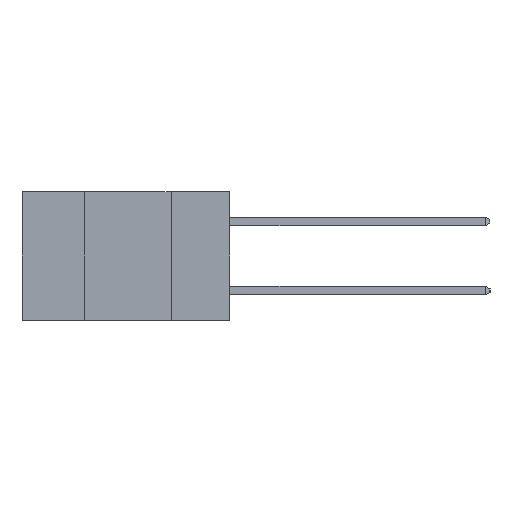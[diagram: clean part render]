
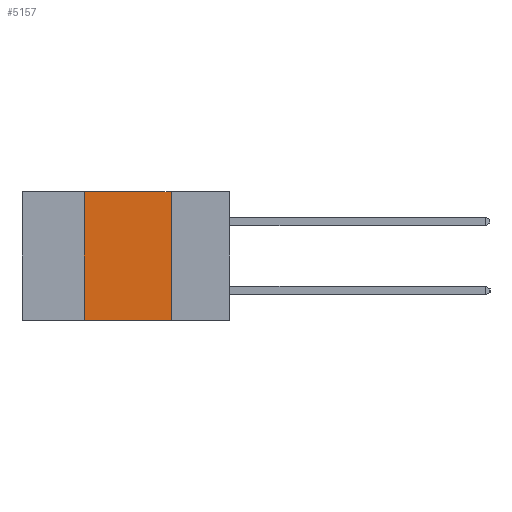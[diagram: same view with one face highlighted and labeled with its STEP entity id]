
A CAD part, left-side view. The second image highlights one B-rep face of the part: STEP entity #5157.
In plain terms, the highlighted planar face has unit normal (-1, 0, 0).
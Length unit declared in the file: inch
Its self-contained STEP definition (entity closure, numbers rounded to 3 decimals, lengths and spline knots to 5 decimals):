
#40 = VERTEX_POINT ( 'NONE', #924 ) ;
#129 = EDGE_LOOP ( 'NONE', ( #3457, #1389, #6023, #1905 ) ) ;
#153 = DIRECTION ( 'NONE',  ( 0., -1., 0. ) ) ;
#199 = EDGE_CURVE ( 'NONE', #40, #6996, #1399, .T. ) ;
#924 = CARTESIAN_POINT ( 'NONE',  ( 0., 0.42, -0.37 ) ) ;
#1389 = ORIENTED_EDGE ( 'NONE', *, *, #9285, .F. ) ;
#1399 = LINE ( 'NONE', #3544, #8061 ) ;
#1658 = FACE_OUTER_BOUND ( 'NONE', #129, .T. ) ;
#1905 = ORIENTED_EDGE ( 'NONE', *, *, #6054, .T. ) ;
#2458 = PLANE ( 'NONE',  #2797 ) ;
#2739 = CARTESIAN_POINT ( 'NONE',  ( 0., 0.17, -0.37 ) ) ;
#2797 = AXIS2_PLACEMENT_3D ( 'NONE', #7676, #8531, #3378 ) ;
#2953 = DIRECTION ( 'NONE',  ( 0., 0., 1. ) ) ;
#3378 = DIRECTION ( 'NONE',  ( 0., 0., -1. ) ) ;
#3457 = ORIENTED_EDGE ( 'NONE', *, *, #4736, .F. ) ;
#3544 = CARTESIAN_POINT ( 'NONE',  ( 0., 0.42, -0.37 ) ) ;
#3731 = CARTESIAN_POINT ( 'NONE',  ( 0., 0.6, -0.37 ) ) ;
#3850 = LINE ( 'NONE', #8376, #10306 ) ;
#4030 = LINE ( 'NONE', #5407, #10489 ) ;
#4540 = DIRECTION ( 'NONE',  ( 0., 0., -1. ) ) ;
#4736 = EDGE_CURVE ( 'NONE', #5844, #9064, #4030, .T. ) ;
#5157 = ADVANCED_FACE ( 'NONE', ( #1658 ), #2458, .F. ) ;
#5407 = CARTESIAN_POINT ( 'NONE',  ( 0., 0.17, -0.37 ) ) ;
#5806 = DIRECTION ( 'NONE',  ( 0., -1., 0. ) ) ;
#5844 = VERTEX_POINT ( 'NONE', #6013 ) ;
#6013 = CARTESIAN_POINT ( 'NONE',  ( 0., 0.17, 0. ) ) ;
#6023 = ORIENTED_EDGE ( 'NONE', *, *, #199, .F. ) ;
#6054 = EDGE_CURVE ( 'NONE', #40, #9064, #10206, .T. ) ;
#6616 = CARTESIAN_POINT ( 'NONE',  ( 0., 0.42, 0. ) ) ;
#6996 = VERTEX_POINT ( 'NONE', #6616 ) ;
#7676 = CARTESIAN_POINT ( 'NONE',  ( 0., 0.6, 0. ) ) ;
#8061 = VECTOR ( 'NONE', #2953, 39.37008 ) ;
#8376 = CARTESIAN_POINT ( 'NONE',  ( 0., 0.6, 0. ) ) ;
#8531 = DIRECTION ( 'NONE',  ( 1., 0., 0. ) ) ;
#9064 = VERTEX_POINT ( 'NONE', #2739 ) ;
#9285 = EDGE_CURVE ( 'NONE', #6996, #5844, #3850, .T. ) ;
#9957 = VECTOR ( 'NONE', #153, 39.37008 ) ;
#10206 = LINE ( 'NONE', #3731, #9957 ) ;
#10306 = VECTOR ( 'NONE', #5806, 39.37008 ) ;
#10489 = VECTOR ( 'NONE', #4540, 39.37008 ) ;
